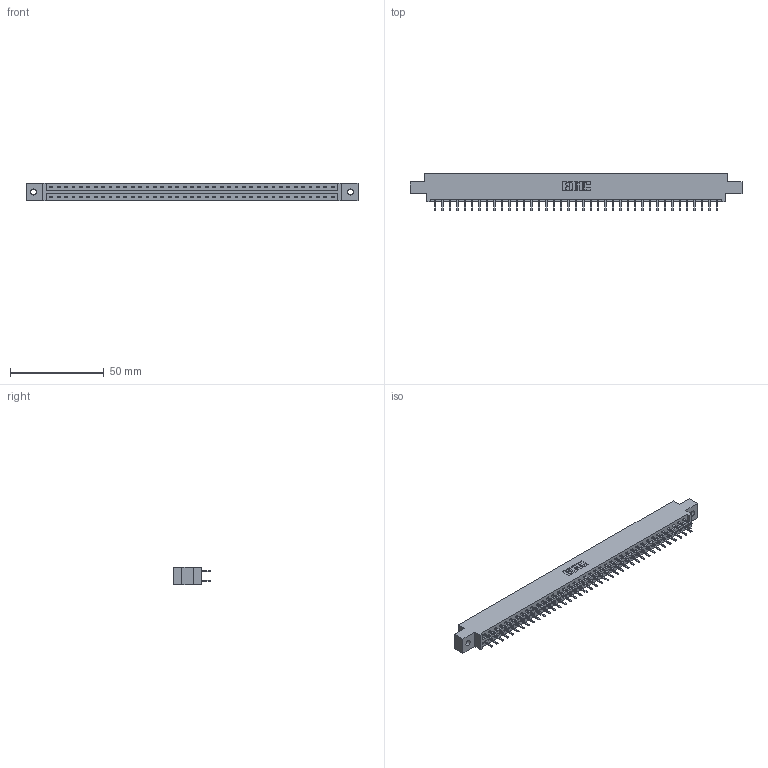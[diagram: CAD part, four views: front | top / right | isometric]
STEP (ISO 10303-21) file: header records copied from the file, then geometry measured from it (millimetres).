
FILE_DESCRIPTION (( 'STEP AP203' ), '1' );
FILE_NAME ('337-078-520-802.STEP', '2018-08-12T15:23:47', ( '' ), ( '' ), 'SwSTEP 2.0', 'SolidWorks 2016', '' );
FILE_SCHEMA (( 'CONFIG_CONTROL_DESIGN' ));
Length unit declared in the file: inch
Products named in the file (3): 345-292-001_345-293-120; 337-078-520-802; 337 Part_0.170 Offset - 0.128 Dia
Assembly tree (79 placements, depth 2):
  337-078-520-802
    337 Part_0.170 Offset - 0.128 Dia
    345-292-001_345-293-120  x78
Bounding box: 177.55 x 20.02 x 9.4 mm (x, y, z)
Volume: 18482.8 mm3; surface area: 20603 mm2
Topology: 79 solids, 79 shells, 4642 faces, 13505 edges, 8794 vertices
Faces by surface type: plane 3194, cylinder 1448
Entity records: 30875 total; most frequent: CARTESIAN_POINT 5218, ORIENTED_EDGE 5142, DIRECTION 4431, EDGE_CURVE 2571, VECTOR 2439, LINE 2439, VERTEX_POINT 1710, AXIS2_PLACEMENT_3D 996
